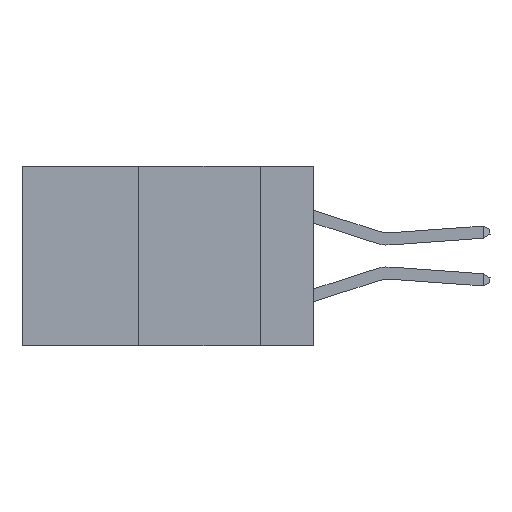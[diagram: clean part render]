
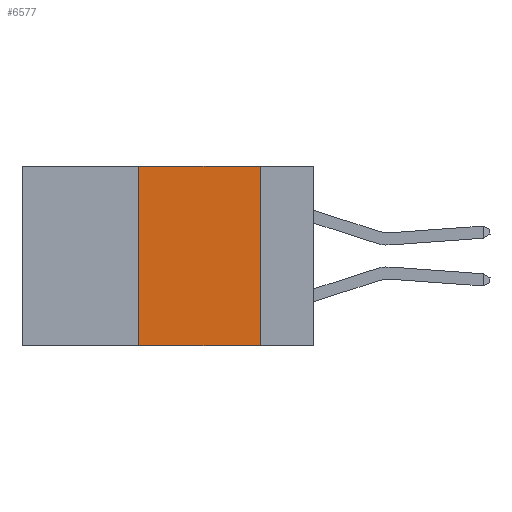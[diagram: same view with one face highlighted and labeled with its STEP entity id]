
A CAD part, left-side view. The second image highlights one B-rep face of the part: STEP entity #6577.
In plain terms, the highlighted planar face has unit normal (-1, 0, 0).
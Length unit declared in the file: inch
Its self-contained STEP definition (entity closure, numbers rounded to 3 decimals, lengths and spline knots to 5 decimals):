
#973 = VERTEX_POINT ( 'NONE', #5920 ) ;
#1748 = CARTESIAN_POINT ( 'NONE',  ( 0., 0.36, -0.37 ) ) ;
#2404 = VECTOR ( 'NONE', #10267, 39.37008 ) ;
#3030 = DIRECTION ( 'NONE',  ( 0., -1., 0. ) ) ;
#4226 = VECTOR ( 'NONE', #11847, 39.37008 ) ;
#4681 = EDGE_LOOP ( 'NONE', ( #26787, #7167, #24387, #23499 ) ) ;
#5920 = CARTESIAN_POINT ( 'NONE',  ( 0., 0.11, -0.37 ) ) ;
#6577 = ADVANCED_FACE ( 'NONE', ( #12341 ), #20034, .F. ) ;
#7167 = ORIENTED_EDGE ( 'NONE', *, *, #26837, .F. ) ;
#7283 = LINE ( 'NONE', #23540, #2404 ) ;
#10267 = DIRECTION ( 'NONE',  ( 0., 0., -1. ) ) ;
#10907 = VERTEX_POINT ( 'NONE', #1748 ) ;
#11370 = CARTESIAN_POINT ( 'NONE',  ( 0., 0.36, 0. ) ) ;
#11406 = EDGE_CURVE ( 'NONE', #11806, #973, #7283, .T. ) ;
#11534 = DIRECTION ( 'NONE',  ( 0., 0., -1. ) ) ;
#11555 = AXIS2_PLACEMENT_3D ( 'NONE', #24442, #20235, #11534 ) ;
#11806 = VERTEX_POINT ( 'NONE', #18192 ) ;
#11847 = DIRECTION ( 'NONE',  ( 0., -1., 0. ) ) ;
#12341 = FACE_OUTER_BOUND ( 'NONE', #4681, .T. ) ;
#12560 = CARTESIAN_POINT ( 'NONE',  ( 0., 0.6, -0.37 ) ) ;
#15214 = VERTEX_POINT ( 'NONE', #25606 ) ;
#15987 = DIRECTION ( 'NONE',  ( 0., 0., 1. ) ) ;
#18192 = CARTESIAN_POINT ( 'NONE',  ( 0., 0.11, 0. ) ) ;
#18407 = LINE ( 'NONE', #11370, #25747 ) ;
#19763 = EDGE_CURVE ( 'NONE', #10907, #973, #21906, .T. ) ;
#20034 = PLANE ( 'NONE',  #11555 ) ;
#20235 = DIRECTION ( 'NONE',  ( 1., 0., 0. ) ) ;
#20578 = CARTESIAN_POINT ( 'NONE',  ( 0., 0.6, 0. ) ) ;
#21906 = LINE ( 'NONE', #12560, #4226 ) ;
#22929 = LINE ( 'NONE', #20578, #23315 ) ;
#23315 = VECTOR ( 'NONE', #3030, 39.37008 ) ;
#23499 = ORIENTED_EDGE ( 'NONE', *, *, #19763, .T. ) ;
#23540 = CARTESIAN_POINT ( 'NONE',  ( 0., 0.11, 0. ) ) ;
#24387 = ORIENTED_EDGE ( 'NONE', *, *, #26572, .F. ) ;
#24442 = CARTESIAN_POINT ( 'NONE',  ( 0., 0.6, 0. ) ) ;
#25606 = CARTESIAN_POINT ( 'NONE',  ( 0., 0.36, 0. ) ) ;
#25747 = VECTOR ( 'NONE', #15987, 39.37008 ) ;
#26572 = EDGE_CURVE ( 'NONE', #10907, #15214, #18407, .T. ) ;
#26787 = ORIENTED_EDGE ( 'NONE', *, *, #11406, .F. ) ;
#26837 = EDGE_CURVE ( 'NONE', #15214, #11806, #22929, .T. ) ;
